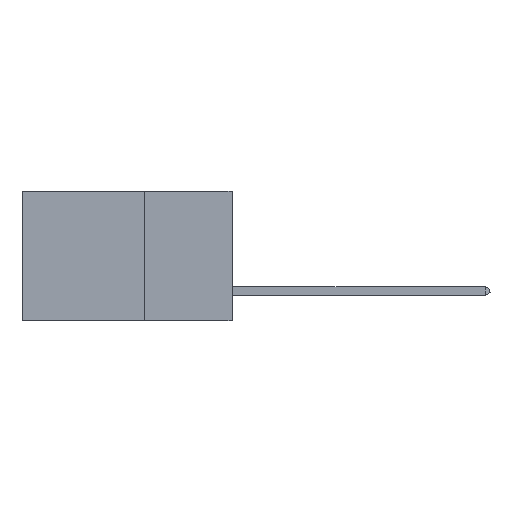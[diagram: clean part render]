
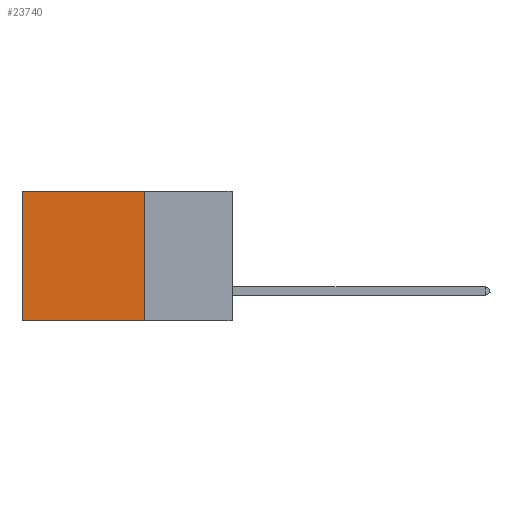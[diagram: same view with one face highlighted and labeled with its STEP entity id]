
A CAD part, left-side view. The second image highlights one B-rep face of the part: STEP entity #23740.
In plain terms, the highlighted planar face has unit normal (-1, 0, 0).
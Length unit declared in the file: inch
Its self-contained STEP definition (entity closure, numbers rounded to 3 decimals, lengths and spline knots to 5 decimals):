
#1770 = CARTESIAN_POINT ( 'NONE',  ( 0.2875, 0.6, 0. ) ) ;
#2300 = DIRECTION ( 'NONE',  ( 1., 0., 0. ) ) ;
#2979 = CARTESIAN_POINT ( 'NONE',  ( 0.2875, 0.25, -0.37 ) ) ;
#7958 = LINE ( 'NONE', #30501, #35693 ) ;
#9636 = VECTOR ( 'NONE', #26198, 39.37008 ) ;
#10052 = CARTESIAN_POINT ( 'NONE',  ( 0.2875, 0.25, 0. ) ) ;
#11099 = EDGE_CURVE ( 'NONE', #11103, #12448, #7958, .T. ) ;
#11103 = VERTEX_POINT ( 'NONE', #12944 ) ;
#12254 = VECTOR ( 'NONE', #15933, 39.37008 ) ;
#12448 = VERTEX_POINT ( 'NONE', #1770 ) ;
#12944 = CARTESIAN_POINT ( 'NONE',  ( 0.2875, 0.25, 0. ) ) ;
#15921 = AXIS2_PLACEMENT_3D ( 'NONE', #10052, #2300, #27585 ) ;
#15933 = DIRECTION ( 'NONE',  ( 0., 1., 0. ) ) ;
#17438 = PLANE ( 'NONE',  #15921 ) ;
#17815 = ORIENTED_EDGE ( 'NONE', *, *, #36094, .T. ) ;
#20556 = VERTEX_POINT ( 'NONE', #2979 ) ;
#21513 = CARTESIAN_POINT ( 'NONE',  ( 0.2875, 0.25, 0. ) ) ;
#23740 = ADVANCED_FACE ( 'NONE', ( #28396 ), #17438, .F. ) ;
#23779 = LINE ( 'NONE', #21513, #9636 ) ;
#25206 = VECTOR ( 'NONE', #26919, 39.37008 ) ;
#25714 = LINE ( 'NONE', #27089, #25206 ) ;
#26198 = DIRECTION ( 'NONE',  ( 0., 0., -1. ) ) ;
#26919 = DIRECTION ( 'NONE',  ( 0., 0., -1. ) ) ;
#27089 = CARTESIAN_POINT ( 'NONE',  ( 0.2875, 0.6, 0. ) ) ;
#27585 = DIRECTION ( 'NONE',  ( 0., 0., -1. ) ) ;
#28396 = FACE_OUTER_BOUND ( 'NONE', #42334, .T. ) ;
#28693 = LINE ( 'NONE', #30974, #12254 ) ;
#30501 = CARTESIAN_POINT ( 'NONE',  ( 0.2875, 0.25, 0. ) ) ;
#30974 = CARTESIAN_POINT ( 'NONE',  ( 0.2875, 0.25, -0.37 ) ) ;
#31319 = ORIENTED_EDGE ( 'NONE', *, *, #33259, .F. ) ;
#32674 = ORIENTED_EDGE ( 'NONE', *, *, #11099, .T. ) ;
#33259 = EDGE_CURVE ( 'NONE', #11103, #20556, #23779, .T. ) ;
#33960 = VERTEX_POINT ( 'NONE', #37530 ) ;
#34581 = DIRECTION ( 'NONE',  ( 0., 1., 0. ) ) ;
#35693 = VECTOR ( 'NONE', #34581, 39.37008 ) ;
#36094 = EDGE_CURVE ( 'NONE', #12448, #33960, #25714, .T. ) ;
#37530 = CARTESIAN_POINT ( 'NONE',  ( 0.2875, 0.6, -0.37 ) ) ;
#40559 = EDGE_CURVE ( 'NONE', #20556, #33960, #28693, .T. ) ;
#42334 = EDGE_LOOP ( 'NONE', ( #17815, #42776, #31319, #32674 ) ) ;
#42776 = ORIENTED_EDGE ( 'NONE', *, *, #40559, .F. ) ;
